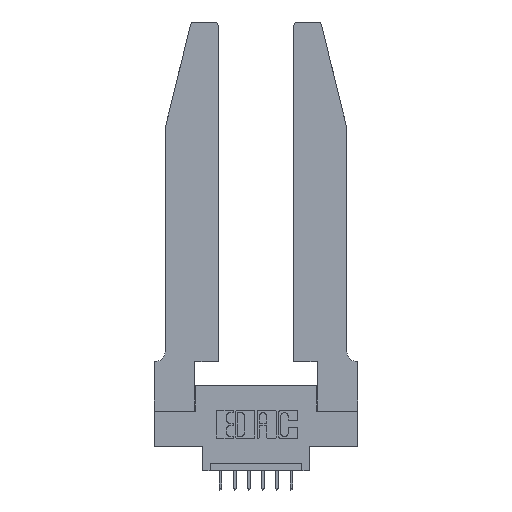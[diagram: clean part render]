
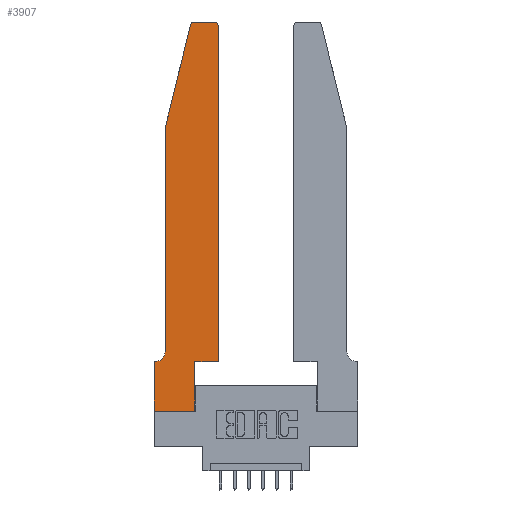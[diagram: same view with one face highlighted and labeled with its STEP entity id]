
A CAD part, top view. The second image highlights one B-rep face of the part: STEP entity #3907.
In plain terms, the highlighted planar face has unit normal (0, 0, 1).
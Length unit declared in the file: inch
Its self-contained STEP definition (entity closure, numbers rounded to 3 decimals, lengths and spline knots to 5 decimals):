
#175 = ORIENTED_EDGE ( 'NONE', *, *, #10169, .T. ) ;
#215 = VERTEX_POINT ( 'NONE', #1945 ) ;
#431 = CARTESIAN_POINT ( 'NONE',  ( 0.0755, 0.35, 0.37 ) ) ;
#629 = EDGE_CURVE ( 'NONE', #215, #12240, #2147, .T. ) ;
#993 = DIRECTION ( 'NONE',  ( 0., 0., 1. ) ) ;
#1021 = CARTESIAN_POINT ( 'NONE',  ( 0., 0.35, 0.37 ) ) ;
#1064 = EDGE_CURVE ( 'NONE', #12240, #3433, #5764, .T. ) ;
#1267 = DIRECTION ( 'NONE',  ( 1., 0., 0. ) ) ;
#1343 = ORIENTED_EDGE ( 'NONE', *, *, #10040, .T. ) ;
#1423 = DIRECTION ( 'NONE',  ( 0., 0., 1. ) ) ;
#1440 = EDGE_LOOP ( 'NONE', ( #10140, #5236, #2747, #9943, #4089, #2831, #9443, #1343, #175, #10391, #9086, #7652 ) ) ;
#1595 = DIRECTION ( 'NONE',  ( -1., 0., 0. ) ) ;
#1945 = CARTESIAN_POINT ( 'NONE',  ( 0.4205, 2.75, 0.37 ) ) ;
#2075 = DIRECTION ( 'NONE',  ( -1., 0., 0. ) ) ;
#2147 = LINE ( 'NONE', #9901, #4339 ) ;
#2187 = DIRECTION ( 'NONE',  ( 0., -1., 0. ) ) ;
#2545 = AXIS2_PLACEMENT_3D ( 'NONE', #12962, #993, #11803 ) ;
#2587 = DIRECTION ( 'NONE',  ( 1., 0., 0. ) ) ;
#2634 = CARTESIAN_POINT ( 'NONE',  ( 0.0055, 0.42, 0.37 ) ) ;
#2705 = VERTEX_POINT ( 'NONE', #3035 ) ;
#2747 = ORIENTED_EDGE ( 'NONE', *, *, #13283, .T. ) ;
#2831 = ORIENTED_EDGE ( 'NONE', *, *, #7472, .T. ) ;
#2924 = CARTESIAN_POINT ( 'NONE',  ( 0.284, 2.75, 0.37 ) ) ;
#2982 = AXIS2_PLACEMENT_3D ( 'NONE', #7920, #5895, #3420 ) ;
#3031 = EDGE_CURVE ( 'NONE', #5551, #215, #8778, .T. ) ;
#3035 = CARTESIAN_POINT ( 'NONE',  ( 0., 0., 0.37 ) ) ;
#3242 = CIRCLE ( 'NONE', #8333, 0.07 ) ;
#3420 = DIRECTION ( 'NONE',  ( 1., 0., 0. ) ) ;
#3433 = VERTEX_POINT ( 'NONE', #14151 ) ;
#3528 = LINE ( 'NONE', #7950, #7895 ) ;
#3655 = VECTOR ( 'NONE', #12066, 39.37008 ) ;
#3691 = CARTESIAN_POINT ( 'NONE',  ( 0.2865, 0.35, 0.37 ) ) ;
#3784 = VERTEX_POINT ( 'NONE', #10652 ) ;
#3832 = VECTOR ( 'NONE', #1595, 39.37008 ) ;
#3907 = ADVANCED_FACE ( 'NONE', ( #4418 ), #5425, .T. ) ;
#4089 = ORIENTED_EDGE ( 'NONE', *, *, #4614, .T. ) ;
#4231 = VERTEX_POINT ( 'NONE', #9261 ) ;
#4339 = VECTOR ( 'NONE', #2075, 39.37008 ) ;
#4418 = FACE_OUTER_BOUND ( 'NONE', #1440, .T. ) ;
#4592 = VERTEX_POINT ( 'NONE', #6624 ) ;
#4614 = EDGE_CURVE ( 'NONE', #6939, #3784, #3242, .T. ) ;
#4859 = AXIS2_PLACEMENT_3D ( 'NONE', #12840, #1423, #2587 ) ;
#4895 = CARTESIAN_POINT ( 'NONE',  ( 0.4505, 2.72, 0.37 ) ) ;
#4898 = DIRECTION ( 'NONE',  ( -1., 0., 0. ) ) ;
#4963 = EDGE_CURVE ( 'NONE', #4231, #4592, #3528, .T. ) ;
#5236 = ORIENTED_EDGE ( 'NONE', *, *, #1064, .T. ) ;
#5425 = PLANE ( 'NONE',  #2545 ) ;
#5551 = VERTEX_POINT ( 'NONE', #4895 ) ;
#5764 = CIRCLE ( 'NONE', #2982, 0.03 ) ;
#5895 = DIRECTION ( 'NONE',  ( 0., 0., 1. ) ) ;
#5987 = DIRECTION ( 'NONE',  ( 0., 0., -1. ) ) ;
#6624 = CARTESIAN_POINT ( 'NONE',  ( 0.4505, 0.35, 0.37 ) ) ;
#6939 = VERTEX_POINT ( 'NONE', #11322 ) ;
#6957 = DIRECTION ( 'NONE',  ( 0., -1., 0. ) ) ;
#7472 = EDGE_CURVE ( 'NONE', #3784, #12338, #10368, .T. ) ;
#7645 = LINE ( 'NONE', #12405, #3655 ) ;
#7652 = ORIENTED_EDGE ( 'NONE', *, *, #3031, .T. ) ;
#7800 = VERTEX_POINT ( 'NONE', #11505 ) ;
#7895 = VECTOR ( 'NONE', #1267, 39.37008 ) ;
#7900 = LINE ( 'NONE', #12456, #13538 ) ;
#7920 = CARTESIAN_POINT ( 'NONE',  ( 0.284, 2.72, 0.37 ) ) ;
#7950 = CARTESIAN_POINT ( 'NONE',  ( 0.4505, 0.35, 0.37 ) ) ;
#8333 = AXIS2_PLACEMENT_3D ( 'NONE', #2634, #5987, #4898 ) ;
#8603 = EDGE_CURVE ( 'NONE', #7800, #6939, #11222, .T. ) ;
#8778 = CIRCLE ( 'NONE', #4859, 0.03 ) ;
#9060 = CARTESIAN_POINT ( 'NONE',  ( 0., 0., 0.37 ) ) ;
#9086 = ORIENTED_EDGE ( 'NONE', *, *, #13861, .T. ) ;
#9203 = LINE ( 'NONE', #9060, #13077 ) ;
#9261 = CARTESIAN_POINT ( 'NONE',  ( 0.2865, 0.35, 0.37 ) ) ;
#9443 = ORIENTED_EDGE ( 'NONE', *, *, #11249, .T. ) ;
#9517 = CARTESIAN_POINT ( 'NONE',  ( 0.2865, 0., 0.37 ) ) ;
#9634 = LINE ( 'NONE', #14054, #10351 ) ;
#9901 = CARTESIAN_POINT ( 'NONE',  ( 0.2605, 2.75, 0.37 ) ) ;
#9943 = ORIENTED_EDGE ( 'NONE', *, *, #8603, .T. ) ;
#10040 = EDGE_CURVE ( 'NONE', #2705, #13978, #7900, .T. ) ;
#10138 = LINE ( 'NONE', #3691, #12142 ) ;
#10140 = ORIENTED_EDGE ( 'NONE', *, *, #629, .T. ) ;
#10169 = EDGE_CURVE ( 'NONE', #13978, #4231, #10138, .T. ) ;
#10351 = VECTOR ( 'NONE', #12808, 39.37008 ) ;
#10358 = DIRECTION ( 'NONE',  ( 1., 0., 0. ) ) ;
#10368 = LINE ( 'NONE', #431, #3832 ) ;
#10391 = ORIENTED_EDGE ( 'NONE', *, *, #4963, .T. ) ;
#10652 = CARTESIAN_POINT ( 'NONE',  ( 0.0055, 0.35, 0.37 ) ) ;
#11222 = LINE ( 'NONE', #14314, #12543 ) ;
#11249 = EDGE_CURVE ( 'NONE', #12338, #2705, #9203, .T. ) ;
#11322 = CARTESIAN_POINT ( 'NONE',  ( 0.0755, 0.42, 0.37 ) ) ;
#11505 = CARTESIAN_POINT ( 'NONE',  ( 0.0755, 2., 0.37 ) ) ;
#11803 = DIRECTION ( 'NONE',  ( 1., 0., 0. ) ) ;
#12066 = DIRECTION ( 'NONE',  ( 0., 1., 0. ) ) ;
#12142 = VECTOR ( 'NONE', #12380, 39.37008 ) ;
#12240 = VERTEX_POINT ( 'NONE', #2924 ) ;
#12338 = VERTEX_POINT ( 'NONE', #1021 ) ;
#12380 = DIRECTION ( 'NONE',  ( 0., 1., 0. ) ) ;
#12405 = CARTESIAN_POINT ( 'NONE',  ( 0.4505, 0.35, 0.37 ) ) ;
#12456 = CARTESIAN_POINT ( 'NONE',  ( 0., 0., 0.37 ) ) ;
#12543 = VECTOR ( 'NONE', #2187, 39.37008 ) ;
#12808 = DIRECTION ( 'NONE',  ( -0.239, -0.971, 0. ) ) ;
#12840 = CARTESIAN_POINT ( 'NONE',  ( 0.4205, 2.72, 0.37 ) ) ;
#12962 = CARTESIAN_POINT ( 'NONE',  ( 0., 0.35, 0.37 ) ) ;
#13077 = VECTOR ( 'NONE', #6957, 39.37008 ) ;
#13283 = EDGE_CURVE ( 'NONE', #3433, #7800, #9634, .T. ) ;
#13538 = VECTOR ( 'NONE', #10358, 39.37008 ) ;
#13861 = EDGE_CURVE ( 'NONE', #4592, #5551, #7645, .T. ) ;
#13978 = VERTEX_POINT ( 'NONE', #9517 ) ;
#14054 = CARTESIAN_POINT ( 'NONE',  ( 0.0755, 2., 0.37 ) ) ;
#14151 = CARTESIAN_POINT ( 'NONE',  ( 0.25487, 2.72718, 0.37 ) ) ;
#14314 = CARTESIAN_POINT ( 'NONE',  ( 0.0755, 2., 0.37 ) ) ;
